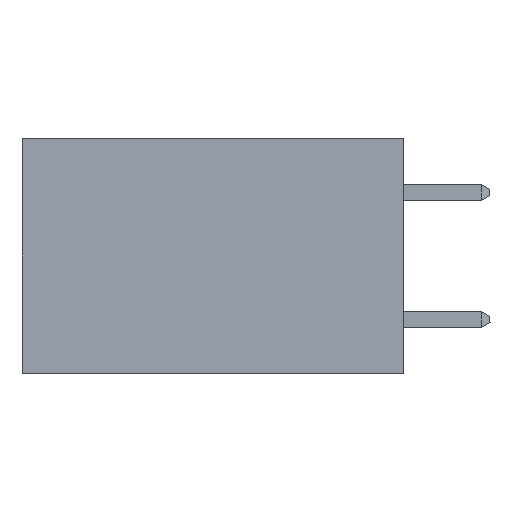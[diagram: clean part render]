
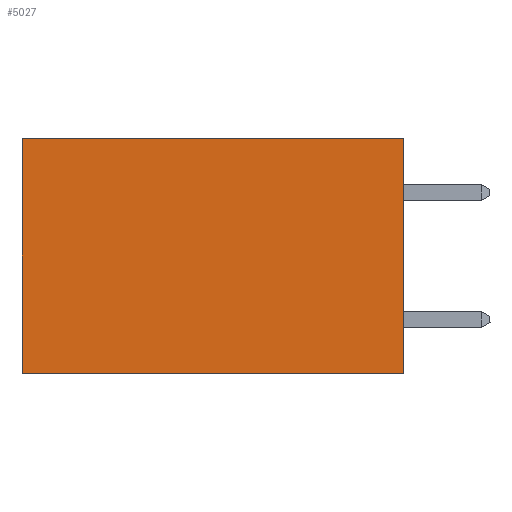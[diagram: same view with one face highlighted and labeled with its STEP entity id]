
A CAD part, left-side view. The second image highlights one B-rep face of the part: STEP entity #5027.
In plain terms, the highlighted planar face has unit normal (-1, 0, 0).
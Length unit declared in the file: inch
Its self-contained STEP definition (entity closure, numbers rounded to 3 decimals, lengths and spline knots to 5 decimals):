
#1104 = DIRECTION ( 'NONE',  ( 0., 0., -1. ) ) ;
#2455 = VECTOR ( 'NONE', #27739, 39.37008 ) ;
#2646 = LINE ( 'NONE', #20409, #5612 ) ;
#2859 = VERTEX_POINT ( 'NONE', #14764 ) ;
#3225 = CARTESIAN_POINT ( 'NONE',  ( 0.2875, 0., 0. ) ) ;
#4202 = CARTESIAN_POINT ( 'NONE',  ( 0.2875, 0., -0.37 ) ) ;
#4318 = VECTOR ( 'NONE', #1104, 39.37008 ) ;
#4481 = LINE ( 'NONE', #30050, #22355 ) ;
#5027 = ADVANCED_FACE ( 'NONE', ( #11889 ), #5393, .F. ) ;
#5040 = LINE ( 'NONE', #21051, #4318 ) ;
#5393 = PLANE ( 'NONE',  #10942 ) ;
#5612 = VECTOR ( 'NONE', #18803, 39.37008 ) ;
#7072 = ORIENTED_EDGE ( 'NONE', *, *, #12271, .T. ) ;
#10942 = AXIS2_PLACEMENT_3D ( 'NONE', #3225, #17195, #28675 ) ;
#11889 = FACE_OUTER_BOUND ( 'NONE', #14698, .T. ) ;
#12271 = EDGE_CURVE ( 'NONE', #2859, #28468, #2646, .T. ) ;
#12497 = VERTEX_POINT ( 'NONE', #29740 ) ;
#13006 = ORIENTED_EDGE ( 'NONE', *, *, #26339, .F. ) ;
#13034 = VERTEX_POINT ( 'NONE', #13099 ) ;
#13099 = CARTESIAN_POINT ( 'NONE',  ( 0.2875, 0., -0.37 ) ) ;
#14698 = EDGE_LOOP ( 'NONE', ( #18374, #13006, #24238, #7072 ) ) ;
#14764 = CARTESIAN_POINT ( 'NONE',  ( 0.2875, 0., 0. ) ) ;
#15145 = EDGE_CURVE ( 'NONE', #28468, #12497, #4481, .T. ) ;
#17195 = DIRECTION ( 'NONE',  ( 1., 0., 0. ) ) ;
#18374 = ORIENTED_EDGE ( 'NONE', *, *, #15145, .T. ) ;
#18675 = CARTESIAN_POINT ( 'NONE',  ( 0.2875, 0.6, 0. ) ) ;
#18803 = DIRECTION ( 'NONE',  ( 0., 1., 0. ) ) ;
#20379 = DIRECTION ( 'NONE',  ( 0., 0., -1. ) ) ;
#20409 = CARTESIAN_POINT ( 'NONE',  ( 0.2875, 0., 0. ) ) ;
#21050 = LINE ( 'NONE', #4202, #2455 ) ;
#21051 = CARTESIAN_POINT ( 'NONE',  ( 0.2875, 0., 0. ) ) ;
#22355 = VECTOR ( 'NONE', #20379, 39.37008 ) ;
#24238 = ORIENTED_EDGE ( 'NONE', *, *, #26051, .F. ) ;
#26051 = EDGE_CURVE ( 'NONE', #2859, #13034, #5040, .T. ) ;
#26339 = EDGE_CURVE ( 'NONE', #13034, #12497, #21050, .T. ) ;
#27739 = DIRECTION ( 'NONE',  ( 0., 1., 0. ) ) ;
#28468 = VERTEX_POINT ( 'NONE', #18675 ) ;
#28675 = DIRECTION ( 'NONE',  ( 0., 0., -1. ) ) ;
#29740 = CARTESIAN_POINT ( 'NONE',  ( 0.2875, 0.6, -0.37 ) ) ;
#30050 = CARTESIAN_POINT ( 'NONE',  ( 0.2875, 0.6, 0. ) ) ;
